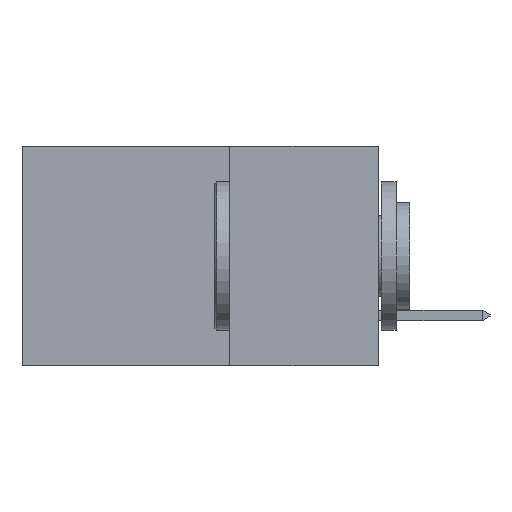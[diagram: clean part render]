
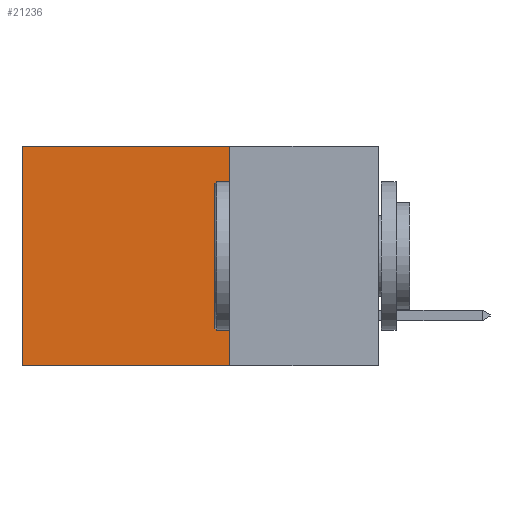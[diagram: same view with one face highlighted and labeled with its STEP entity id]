
A CAD part, left-side view. The second image highlights one B-rep face of the part: STEP entity #21236.
In plain terms, the highlighted planar face has unit normal (-1, 0, 0).
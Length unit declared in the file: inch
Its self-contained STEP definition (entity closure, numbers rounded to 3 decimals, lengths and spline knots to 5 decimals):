
#823 = FACE_OUTER_BOUND ( 'NONE', #14962, .T. ) ;
#1043 = CARTESIAN_POINT ( 'NONE',  ( 0.298, 0.25, 0. ) ) ;
#1348 = CARTESIAN_POINT ( 'NONE',  ( 0.298, 0.25, 0. ) ) ;
#2010 = VECTOR ( 'NONE', #4430, 39.37008 ) ;
#2936 = ORIENTED_EDGE ( 'NONE', *, *, #14442, .T. ) ;
#2996 = LINE ( 'NONE', #13389, #13037 ) ;
#3076 = AXIS2_PLACEMENT_3D ( 'NONE', #1348, #14826, #4726 ) ;
#3158 = VERTEX_POINT ( 'NONE', #17864 ) ;
#3541 = VECTOR ( 'NONE', #16522, 39.37008 ) ;
#4430 = DIRECTION ( 'NONE',  ( 0., 1., 0. ) ) ;
#4726 = DIRECTION ( 'NONE',  ( 0., 0., -1. ) ) ;
#6598 = CARTESIAN_POINT ( 'NONE',  ( 0.298, 0.25, -0.37 ) ) ;
#7025 = LINE ( 'NONE', #1043, #2010 ) ;
#8027 = VERTEX_POINT ( 'NONE', #6598 ) ;
#8288 = DIRECTION ( 'NONE',  ( 0., 1., 0. ) ) ;
#8873 = ORIENTED_EDGE ( 'NONE', *, *, #18420, .F. ) ;
#9066 = CARTESIAN_POINT ( 'NONE',  ( 0.298, 0.25, 0. ) ) ;
#9983 = ORIENTED_EDGE ( 'NONE', *, *, #15737, .F. ) ;
#10745 = DIRECTION ( 'NONE',  ( 0., 0., -1. ) ) ;
#11193 = VERTEX_POINT ( 'NONE', #13738 ) ;
#11449 = PLANE ( 'NONE',  #3076 ) ;
#11497 = CARTESIAN_POINT ( 'NONE',  ( 0.298, 0.6, 0. ) ) ;
#13037 = VECTOR ( 'NONE', #8288, 39.37008 ) ;
#13389 = CARTESIAN_POINT ( 'NONE',  ( 0.298, 0.25, -0.37 ) ) ;
#13738 = CARTESIAN_POINT ( 'NONE',  ( 0.298, 0.6, 0. ) ) ;
#14138 = VECTOR ( 'NONE', #10745, 39.37008 ) ;
#14442 = EDGE_CURVE ( 'NONE', #3158, #11193, #7025, .T. ) ;
#14651 = LINE ( 'NONE', #9066, #14138 ) ;
#14826 = DIRECTION ( 'NONE',  ( 1., 0., 0. ) ) ;
#14962 = EDGE_LOOP ( 'NONE', ( #17230, #9983, #8873, #2936 ) ) ;
#15233 = EDGE_CURVE ( 'NONE', #11193, #17126, #21203, .T. ) ;
#15455 = CARTESIAN_POINT ( 'NONE',  ( 0.298, 0.6, -0.37 ) ) ;
#15737 = EDGE_CURVE ( 'NONE', #8027, #17126, #2996, .T. ) ;
#16522 = DIRECTION ( 'NONE',  ( 0., 0., -1. ) ) ;
#17126 = VERTEX_POINT ( 'NONE', #15455 ) ;
#17230 = ORIENTED_EDGE ( 'NONE', *, *, #15233, .T. ) ;
#17864 = CARTESIAN_POINT ( 'NONE',  ( 0.298, 0.25, 0. ) ) ;
#18420 = EDGE_CURVE ( 'NONE', #3158, #8027, #14651, .T. ) ;
#21203 = LINE ( 'NONE', #11497, #3541 ) ;
#21236 = ADVANCED_FACE ( 'NONE', ( #823 ), #11449, .F. ) ;
